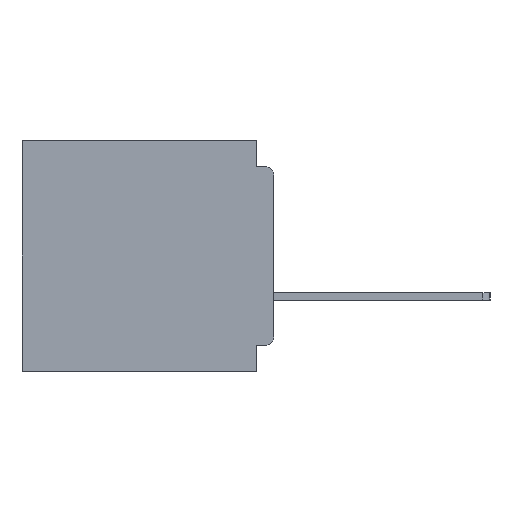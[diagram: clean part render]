
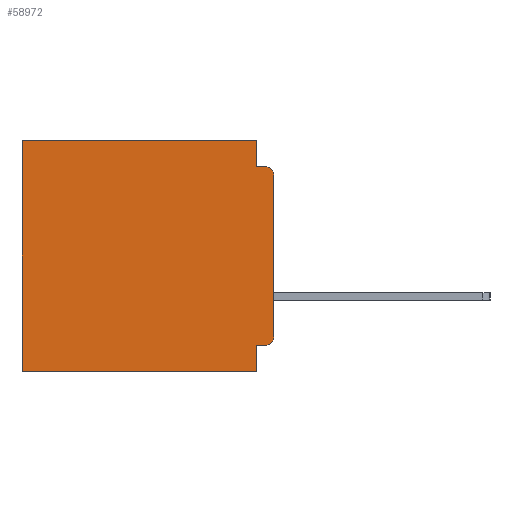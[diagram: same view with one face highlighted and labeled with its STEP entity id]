
A CAD part, left-side view. The second image highlights one B-rep face of the part: STEP entity #58972.
In plain terms, the highlighted planar face has unit normal (-1, 0, 0).
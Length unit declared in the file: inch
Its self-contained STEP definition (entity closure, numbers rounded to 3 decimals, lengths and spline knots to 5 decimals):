
#81 = CARTESIAN_POINT ( 'NONE',  ( 0.3, 0., -0.4 ) ) ;
#497 = DIRECTION ( 'NONE',  ( 0., 0., -1. ) ) ;
#692 = LINE ( 'NONE', #81, #27023 ) ;
#2405 = LINE ( 'NONE', #21873, #28695 ) ;
#2743 = LINE ( 'NONE', #2875, #58717 ) ;
#2875 = CARTESIAN_POINT ( 'NONE',  ( 0.3, 0.031, 0. ) ) ;
#2929 = CARTESIAN_POINT ( 'NONE',  ( 0.3, 0.437, 0. ) ) ;
#3395 = EDGE_CURVE ( 'NONE', #35504, #55881, #56977, .T. ) ;
#7164 = AXIS2_PLACEMENT_3D ( 'NONE', #39606, #8021, #44907 ) ;
#7768 = CARTESIAN_POINT ( 'NONE',  ( 0.3, 0.437, -0.4 ) ) ;
#7943 = EDGE_CURVE ( 'NONE', #57633, #33861, #2743, .T. ) ;
#8021 = DIRECTION ( 'NONE',  ( -1., 0., 0. ) ) ;
#8073 = DIRECTION ( 'NONE',  ( 1., 0., 0. ) ) ;
#8932 = EDGE_CURVE ( 'NONE', #45873, #51300, #65104, .T. ) ;
#9592 = ORIENTED_EDGE ( 'NONE', *, *, #34180, .F. ) ;
#9985 = VERTEX_POINT ( 'NONE', #45997 ) ;
#10397 = DIRECTION ( 'NONE',  ( 0., 1., 0. ) ) ;
#10510 = EDGE_CURVE ( 'NONE', #30743, #9985, #2405, .T. ) ;
#10638 = CARTESIAN_POINT ( 'NONE',  ( 0.3, 0., -0.34 ) ) ;
#12214 = EDGE_CURVE ( 'NONE', #35504, #29870, #54861, .T. ) ;
#12729 = CARTESIAN_POINT ( 'NONE',  ( 0.3, 0., -0.4 ) ) ;
#13533 = AXIS2_PLACEMENT_3D ( 'NONE', #55728, #8073, #29451 ) ;
#15042 = ORIENTED_EDGE ( 'NONE', *, *, #10510, .F. ) ;
#15696 = CARTESIAN_POINT ( 'NONE',  ( 0.3, 0., 0. ) ) ;
#17346 = DIRECTION ( 'NONE',  ( 0., 0., -1. ) ) ;
#17999 = FACE_OUTER_BOUND ( 'NONE', #51742, .T. ) ;
#20326 = ORIENTED_EDGE ( 'NONE', *, *, #12214, .T. ) ;
#21291 = CARTESIAN_POINT ( 'NONE',  ( 0.3, 0.031, -0.045 ) ) ;
#21405 = CARTESIAN_POINT ( 'NONE',  ( 0.3, 0., -0.045 ) ) ;
#21873 = CARTESIAN_POINT ( 'NONE',  ( 0.3, 0.031, -0.4 ) ) ;
#24706 = DIRECTION ( 'NONE',  ( 0., 1., 0. ) ) ;
#26408 = DIRECTION ( 'NONE',  ( 0., 0., -1. ) ) ;
#26588 = CARTESIAN_POINT ( 'NONE',  ( 0.3, 0.031, -0.355 ) ) ;
#27023 = VECTOR ( 'NONE', #31594, 39.37008 ) ;
#27279 = VECTOR ( 'NONE', #17346, 39.37008 ) ;
#28695 = VECTOR ( 'NONE', #58699, 39.37008 ) ;
#29451 = DIRECTION ( 'NONE',  ( 0., 0., -1. ) ) ;
#29870 = VERTEX_POINT ( 'NONE', #34810 ) ;
#30743 = VERTEX_POINT ( 'NONE', #26588 ) ;
#31046 = ORIENTED_EDGE ( 'NONE', *, *, #54977, .T. ) ;
#31594 = DIRECTION ( 'NONE',  ( 0., 1., 0. ) ) ;
#32020 = DIRECTION ( 'NONE',  ( -1., 0., 0. ) ) ;
#33548 = ORIENTED_EDGE ( 'NONE', *, *, #7943, .F. ) ;
#33861 = VERTEX_POINT ( 'NONE', #21291 ) ;
#34180 = EDGE_CURVE ( 'NONE', #62890, #30743, #47826, .T. ) ;
#34810 = CARTESIAN_POINT ( 'NONE',  ( 0.3, 0.015, -0.045 ) ) ;
#35504 = VERTEX_POINT ( 'NONE', #53747 ) ;
#35968 = CARTESIAN_POINT ( 'NONE',  ( 0.3, 0.031, 0. ) ) ;
#37220 = LINE ( 'NONE', #15696, #63423 ) ;
#37634 = CIRCLE ( 'NONE', #7164, 0.015 ) ;
#39606 = CARTESIAN_POINT ( 'NONE',  ( 0.3, 0.015, -0.34 ) ) ;
#39743 = DIRECTION ( 'NONE',  ( 0., 0., -1. ) ) ;
#39839 = CARTESIAN_POINT ( 'NONE',  ( 0.3, 0.015, -0.355 ) ) ;
#41321 = ORIENTED_EDGE ( 'NONE', *, *, #3395, .F. ) ;
#44426 = ORIENTED_EDGE ( 'NONE', *, *, #66889, .F. ) ;
#44907 = DIRECTION ( 'NONE',  ( 0., 0., -1. ) ) ;
#45873 = VERTEX_POINT ( 'NONE', #2929 ) ;
#45997 = CARTESIAN_POINT ( 'NONE',  ( 0.3, 0.031, -0.4 ) ) ;
#47702 = CARTESIAN_POINT ( 'NONE',  ( 0.3, 0.437, -0.4 ) ) ;
#47816 = ORIENTED_EDGE ( 'NONE', *, *, #8932, .T. ) ;
#47826 = LINE ( 'NONE', #51038, #60054 ) ;
#47846 = ORIENTED_EDGE ( 'NONE', *, *, #62510, .T. ) ;
#49367 = AXIS2_PLACEMENT_3D ( 'NONE', #63457, #32020, #497 ) ;
#51038 = CARTESIAN_POINT ( 'NONE',  ( 0.3, 0., -0.355 ) ) ;
#51300 = VERTEX_POINT ( 'NONE', #7768 ) ;
#51742 = EDGE_LOOP ( 'NONE', ( #41321, #20326, #64648, #33548, #47846, #47816, #44426, #15042, #9592, #31046 ) ) ;
#53747 = CARTESIAN_POINT ( 'NONE',  ( 0.3, 0., -0.06 ) ) ;
#54733 = EDGE_CURVE ( 'NONE', #33861, #29870, #55775, .T. ) ;
#54861 = CIRCLE ( 'NONE', #49367, 0.015 ) ;
#54977 = EDGE_CURVE ( 'NONE', #62890, #55881, #37634, .T. ) ;
#55728 = CARTESIAN_POINT ( 'NONE',  ( 0.3, 0., -0.4 ) ) ;
#55775 = LINE ( 'NONE', #21405, #66274 ) ;
#55881 = VERTEX_POINT ( 'NONE', #10638 ) ;
#56977 = LINE ( 'NONE', #12729, #27279 ) ;
#57633 = VERTEX_POINT ( 'NONE', #35968 ) ;
#58699 = DIRECTION ( 'NONE',  ( 0., 0., -1. ) ) ;
#58717 = VECTOR ( 'NONE', #39743, 39.37008 ) ;
#58972 = ADVANCED_FACE ( 'NONE', ( #17999 ), #60938, .F. ) ;
#60054 = VECTOR ( 'NONE', #24706, 39.37008 ) ;
#60938 = PLANE ( 'NONE',  #13533 ) ;
#62510 = EDGE_CURVE ( 'NONE', #57633, #45873, #37220, .T. ) ;
#62890 = VERTEX_POINT ( 'NONE', #39839 ) ;
#63412 = DIRECTION ( 'NONE',  ( 0., -1., 0. ) ) ;
#63423 = VECTOR ( 'NONE', #10397, 39.37008 ) ;
#63457 = CARTESIAN_POINT ( 'NONE',  ( 0.3, 0.015, -0.06 ) ) ;
#63521 = VECTOR ( 'NONE', #26408, 39.37008 ) ;
#64648 = ORIENTED_EDGE ( 'NONE', *, *, #54733, .F. ) ;
#65104 = LINE ( 'NONE', #47702, #63521 ) ;
#66274 = VECTOR ( 'NONE', #63412, 39.37008 ) ;
#66889 = EDGE_CURVE ( 'NONE', #9985, #51300, #692, .T. ) ;
